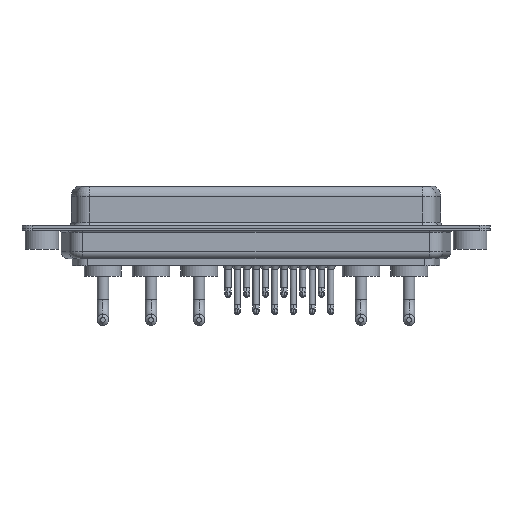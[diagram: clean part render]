
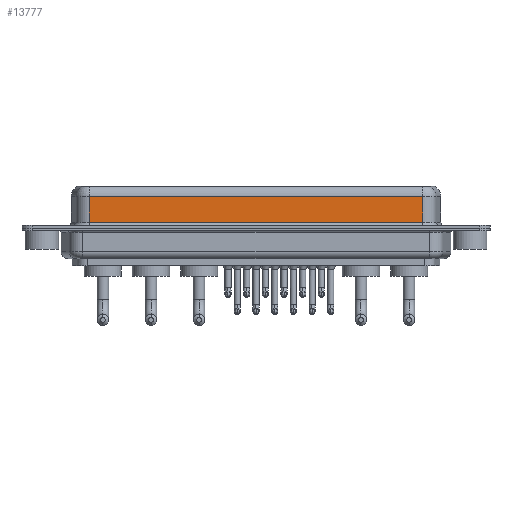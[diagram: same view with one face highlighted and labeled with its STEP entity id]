
A CAD part, front view. The second image highlights one B-rep face of the part: STEP entity #13777.
In plain terms, the highlighted planar face has unit normal (0, -1, 0).
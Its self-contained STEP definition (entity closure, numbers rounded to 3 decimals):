
#85 = CARTESIAN_POINT ( 'NONE',  ( 56.462, -3.95, 4.65 ) ) ;
#644 = VECTOR ( 'NONE', #19856, 1000. ) ;
#1338 = VERTEX_POINT ( 'NONE', #14702 ) ;
#1829 = CARTESIAN_POINT ( 'NONE',  ( 56.462, -3.95, 6.4 ) ) ;
#2360 = EDGE_CURVE ( 'NONE', #6462, #5716, #19651, .T. ) ;
#4458 = DIRECTION ( 'NONE',  ( 1., 0., 0. ) ) ;
#4480 = ORIENTED_EDGE ( 'NONE', *, *, #14556, .T. ) ;
#4653 = CARTESIAN_POINT ( 'NONE',  ( 56.462, -3.95, 4.65 ) ) ;
#5215 = DIRECTION ( 'NONE',  ( 0., 0., 1. ) ) ;
#5541 = EDGE_CURVE ( 'NONE', #18284, #1338, #8387, .T. ) ;
#5716 = VERTEX_POINT ( 'NONE', #17087 ) ;
#6462 = VERTEX_POINT ( 'NONE', #13987 ) ;
#7505 = ORIENTED_EDGE ( 'NONE', *, *, #2360, .T. ) ;
#8040 = LINE ( 'NONE', #4653, #15049 ) ;
#8295 = DIRECTION ( 'NONE',  ( 0., 1., 0. ) ) ;
#8387 = LINE ( 'NONE', #14648, #13162 ) ;
#9686 = DIRECTION ( 'NONE',  ( -1., 0., 0. ) ) ;
#11659 = DIRECTION ( 'NONE',  ( 0., 0., -1. ) ) ;
#11788 = AXIS2_PLACEMENT_3D ( 'NONE', #1829, #8295, #5215 ) ;
#13162 = VECTOR ( 'NONE', #11659, 1000. ) ;
#13368 = EDGE_CURVE ( 'NONE', #18284, #6462, #8040, .T. ) ;
#13777 = ADVANCED_FACE ( 'NONE', ( #19171 ), #17634, .F. ) ;
#13987 = CARTESIAN_POINT ( 'NONE',  ( 7.038, -3.95, 4.65 ) ) ;
#13998 = LINE ( 'NONE', #20263, #19345 ) ;
#14556 = EDGE_CURVE ( 'NONE', #5716, #1338, #13998, .T. ) ;
#14648 = CARTESIAN_POINT ( 'NONE',  ( 56.462, -3.95, 6.4 ) ) ;
#14702 = CARTESIAN_POINT ( 'NONE',  ( 56.462, -3.95, 0.9 ) ) ;
#15049 = VECTOR ( 'NONE', #9686, 1000. ) ;
#15968 = ORIENTED_EDGE ( 'NONE', *, *, #13368, .T. ) ;
#16567 = CARTESIAN_POINT ( 'NONE',  ( 7.038, -3.95, 6.4 ) ) ;
#16581 = ORIENTED_EDGE ( 'NONE', *, *, #5541, .F. ) ;
#17087 = CARTESIAN_POINT ( 'NONE',  ( 7.038, -3.95, 0.9 ) ) ;
#17405 = EDGE_LOOP ( 'NONE', ( #16581, #15968, #7505, #4480 ) ) ;
#17634 = PLANE ( 'NONE',  #11788 ) ;
#18284 = VERTEX_POINT ( 'NONE', #85 ) ;
#19171 = FACE_OUTER_BOUND ( 'NONE', #17405, .T. ) ;
#19345 = VECTOR ( 'NONE', #4458, 1000. ) ;
#19651 = LINE ( 'NONE', #16567, #644 ) ;
#19856 = DIRECTION ( 'NONE',  ( 0., 0., -1. ) ) ;
#20263 = CARTESIAN_POINT ( 'NONE',  ( 56.462, -3.95, 0.9 ) ) ;
